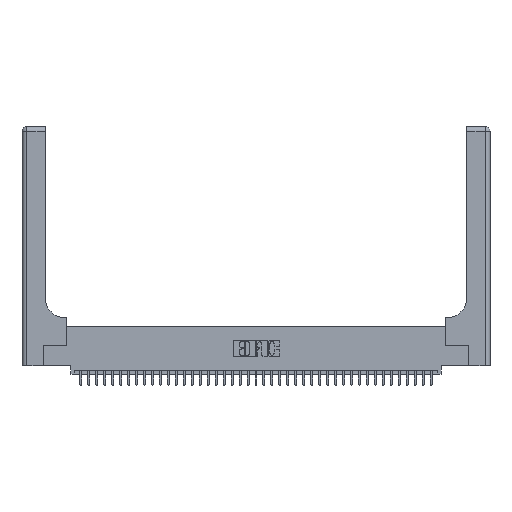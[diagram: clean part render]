
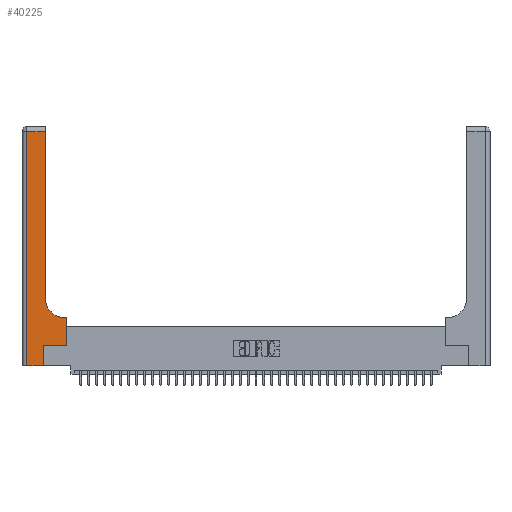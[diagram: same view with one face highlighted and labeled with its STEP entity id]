
A CAD part, top view. The second image highlights one B-rep face of the part: STEP entity #40225.
In plain terms, the highlighted planar face has unit normal (0, 0, 1).
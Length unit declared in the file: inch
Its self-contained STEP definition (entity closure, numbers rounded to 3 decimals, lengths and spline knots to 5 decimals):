
#206 = LINE ( 'NONE', #26878, #8498 ) ;
#730 = VECTOR ( 'NONE', #9378, 39.37008 ) ;
#746 = ORIENTED_EDGE ( 'NONE', *, *, #3004, .T. ) ;
#1664 = EDGE_CURVE ( 'NONE', #33698, #5833, #23679, .T. ) ;
#2492 = ORIENTED_EDGE ( 'NONE', *, *, #1664, .T. ) ;
#2989 = CARTESIAN_POINT ( 'NONE',  ( 0.06, 2.94, 0.37 ) ) ;
#3004 = EDGE_CURVE ( 'NONE', #20327, #24447, #25545, .T. ) ;
#3357 = DIRECTION ( 'NONE',  ( 0., 0., -1. ) ) ;
#3628 = VECTOR ( 'NONE', #36495, 39.37008 ) ;
#4216 = ORIENTED_EDGE ( 'NONE', *, *, #33342, .T. ) ;
#4961 = CARTESIAN_POINT ( 'NONE',  ( 0.269, 0.25, 0.37 ) ) ;
#5027 = DIRECTION ( 'NONE',  ( -1., 0., 0. ) ) ;
#5146 = DIRECTION ( 'NONE',  ( 0., 1., 0. ) ) ;
#5833 = VERTEX_POINT ( 'NONE', #35082 ) ;
#5989 = EDGE_CURVE ( 'NONE', #18411, #35851, #23800, .T. ) ;
#7831 = ORIENTED_EDGE ( 'NONE', *, *, #29513, .T. ) ;
#8356 = VERTEX_POINT ( 'NONE', #30842 ) ;
#8385 = CARTESIAN_POINT ( 'NONE',  ( 0.06, 0., 0.37 ) ) ;
#8465 = CARTESIAN_POINT ( 'NONE',  ( 0.2915, 3., 0.37 ) ) ;
#8498 = VECTOR ( 'NONE', #5146, 39.37008 ) ;
#8521 = VECTOR ( 'NONE', #30432, 39.37008 ) ;
#9308 = CARTESIAN_POINT ( 'NONE',  ( 0.269, 0., 0.37 ) ) ;
#9378 = DIRECTION ( 'NONE',  ( -1., 0., 0. ) ) ;
#9496 = LINE ( 'NONE', #27295, #8521 ) ;
#11099 = CARTESIAN_POINT ( 'NONE',  ( 0., 3., 0.37 ) ) ;
#11830 = LINE ( 'NONE', #8465, #3628 ) ;
#12530 = EDGE_CURVE ( 'NONE', #35851, #8356, #206, .T. ) ;
#12761 = CARTESIAN_POINT ( 'NONE',  ( 0.5585, 0.6, 0.37 ) ) ;
#13052 = FACE_OUTER_BOUND ( 'NONE', #38080, .T. ) ;
#14107 = EDGE_CURVE ( 'NONE', #24447, #18411, #39078, .T. ) ;
#15026 = DIRECTION ( 'NONE',  ( 0., -1., 0. ) ) ;
#15106 = LINE ( 'NONE', #4961, #29793 ) ;
#15349 = VERTEX_POINT ( 'NONE', #18557 ) ;
#15490 = VECTOR ( 'NONE', #39227, 39.37008 ) ;
#16465 = ORIENTED_EDGE ( 'NONE', *, *, #5989, .T. ) ;
#18411 = VERTEX_POINT ( 'NONE', #8385 ) ;
#18557 = CARTESIAN_POINT ( 'NONE',  ( 0.5585, 0.25, 0.37 ) ) ;
#18974 = DIRECTION ( 'NONE',  ( -1., 0., 0. ) ) ;
#20327 = VERTEX_POINT ( 'NONE', #38664 ) ;
#20356 = ORIENTED_EDGE ( 'NONE', *, *, #33620, .T. ) ;
#21543 = AXIS2_PLACEMENT_3D ( 'NONE', #11099, #23560, #5027 ) ;
#21848 = CARTESIAN_POINT ( 'NONE',  ( 0.5415, 0.85, 0.37 ) ) ;
#23560 = DIRECTION ( 'NONE',  ( 0., 0., -1. ) ) ;
#23679 = CIRCLE ( 'NONE', #27241, 0.25 ) ;
#23800 = LINE ( 'NONE', #36152, #15490 ) ;
#24345 = EDGE_CURVE ( 'NONE', #15349, #28185, #9496, .T. ) ;
#24447 = VERTEX_POINT ( 'NONE', #2989 ) ;
#25020 = DIRECTION ( 'NONE',  ( 1., 0., 0. ) ) ;
#25493 = VECTOR ( 'NONE', #15026, 39.37008 ) ;
#25545 = LINE ( 'NONE', #27919, #730 ) ;
#25577 = CARTESIAN_POINT ( 'NONE',  ( 0.5415, 0.6, 0.37 ) ) ;
#26878 = CARTESIAN_POINT ( 'NONE',  ( 0.269, 0., 0.37 ) ) ;
#27241 = AXIS2_PLACEMENT_3D ( 'NONE', #21848, #3357, #25020 ) ;
#27295 = CARTESIAN_POINT ( 'NONE',  ( 0.5585, 0.25, 0.37 ) ) ;
#27919 = CARTESIAN_POINT ( 'NONE',  ( 0., 2.94, 0.37 ) ) ;
#28185 = VERTEX_POINT ( 'NONE', #12761 ) ;
#28332 = CARTESIAN_POINT ( 'NONE',  ( 0.2915, 0.6, 0.37 ) ) ;
#29513 = EDGE_CURVE ( 'NONE', #8356, #15349, #15106, .T. ) ;
#29793 = VECTOR ( 'NONE', #39133, 39.37008 ) ;
#30432 = DIRECTION ( 'NONE',  ( 0., 1., 0. ) ) ;
#30842 = CARTESIAN_POINT ( 'NONE',  ( 0.269, 0.25, 0.37 ) ) ;
#32869 = PLANE ( 'NONE',  #21543 ) ;
#33251 = VECTOR ( 'NONE', #18974, 39.37008 ) ;
#33342 = EDGE_CURVE ( 'NONE', #5833, #20327, #11830, .T. ) ;
#33620 = EDGE_CURVE ( 'NONE', #28185, #33698, #34224, .T. ) ;
#33647 = ORIENTED_EDGE ( 'NONE', *, *, #24345, .T. ) ;
#33698 = VERTEX_POINT ( 'NONE', #25577 ) ;
#33730 = CARTESIAN_POINT ( 'NONE',  ( 0.06, 3., 0.37 ) ) ;
#34224 = LINE ( 'NONE', #28332, #33251 ) ;
#35082 = CARTESIAN_POINT ( 'NONE',  ( 0.2915, 0.85, 0.37 ) ) ;
#35851 = VERTEX_POINT ( 'NONE', #9308 ) ;
#36066 = ORIENTED_EDGE ( 'NONE', *, *, #12530, .T. ) ;
#36152 = CARTESIAN_POINT ( 'NONE',  ( 0., 0., 0.37 ) ) ;
#36320 = ORIENTED_EDGE ( 'NONE', *, *, #14107, .T. ) ;
#36495 = DIRECTION ( 'NONE',  ( 0., 1., 0. ) ) ;
#38080 = EDGE_LOOP ( 'NONE', ( #4216, #746, #36320, #16465, #36066, #7831, #33647, #20356, #2492 ) ) ;
#38664 = CARTESIAN_POINT ( 'NONE',  ( 0.2915, 2.94, 0.37 ) ) ;
#39078 = LINE ( 'NONE', #33730, #25493 ) ;
#39133 = DIRECTION ( 'NONE',  ( 1., 0., 0. ) ) ;
#39227 = DIRECTION ( 'NONE',  ( 1., 0., 0. ) ) ;
#40225 = ADVANCED_FACE ( 'NONE', ( #13052 ), #32869, .F. ) ;
